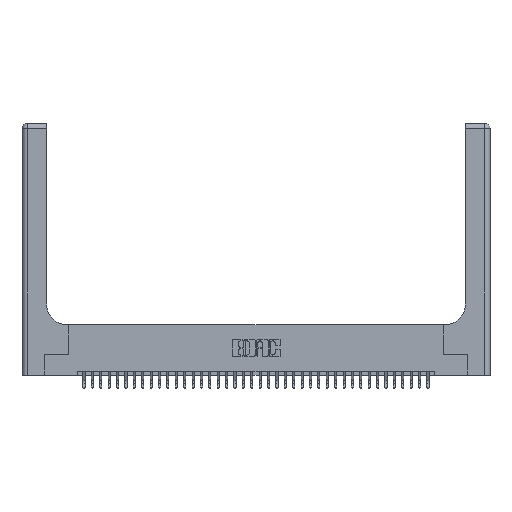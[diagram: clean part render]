
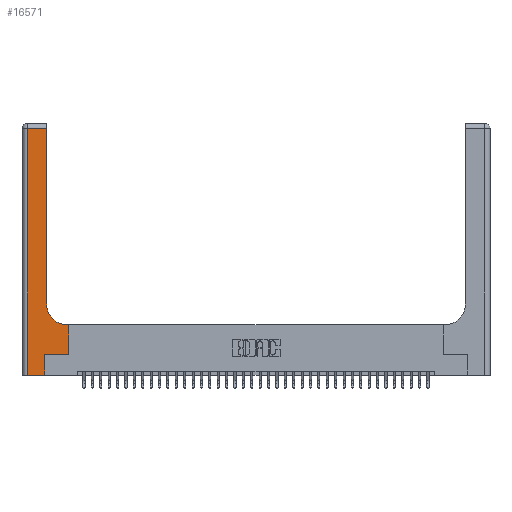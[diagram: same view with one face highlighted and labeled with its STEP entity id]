
A CAD part, top view. The second image highlights one B-rep face of the part: STEP entity #16571.
In plain terms, the highlighted planar face has unit normal (0, 0, 1).
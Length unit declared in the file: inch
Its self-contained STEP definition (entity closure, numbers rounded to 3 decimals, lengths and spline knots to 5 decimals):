
#572 = ORIENTED_EDGE ( 'NONE', *, *, #17456, .T. ) ;
#1190 = CARTESIAN_POINT ( 'NONE',  ( 0.5415, 0.6, 0.37 ) ) ;
#1477 = ORIENTED_EDGE ( 'NONE', *, *, #24891, .T. ) ;
#1787 = VERTEX_POINT ( 'NONE', #2523 ) ;
#2523 = CARTESIAN_POINT ( 'NONE',  ( 0.269, 0.25, 0.37 ) ) ;
#2526 = CARTESIAN_POINT ( 'NONE',  ( 0.2915, 3., 0.37 ) ) ;
#2559 = VERTEX_POINT ( 'NONE', #15699 ) ;
#3589 = DIRECTION ( 'NONE',  ( -1., 0., 0. ) ) ;
#4017 = VERTEX_POINT ( 'NONE', #8633 ) ;
#4109 = CARTESIAN_POINT ( 'NONE',  ( 0., 2.94, 0.37 ) ) ;
#5986 = LINE ( 'NONE', #30661, #36426 ) ;
#6241 = CARTESIAN_POINT ( 'NONE',  ( 0.5585, 0.6, 0.37 ) ) ;
#7123 = DIRECTION ( 'NONE',  ( -1., 0., 0. ) ) ;
#7644 = VECTOR ( 'NONE', #7123, 39.37008 ) ;
#7883 = DIRECTION ( 'NONE',  ( 1., 0., 0. ) ) ;
#7961 = LINE ( 'NONE', #22802, #38336 ) ;
#8111 = DIRECTION ( 'NONE',  ( 0., 0., -1. ) ) ;
#8420 = DIRECTION ( 'NONE',  ( 1., 0., 0. ) ) ;
#8490 = CARTESIAN_POINT ( 'NONE',  ( 0.5585, 0.25, 0.37 ) ) ;
#8607 = ORIENTED_EDGE ( 'NONE', *, *, #38312, .T. ) ;
#8633 = CARTESIAN_POINT ( 'NONE',  ( 0.06, 2.94, 0.37 ) ) ;
#9130 = EDGE_CURVE ( 'NONE', #36194, #2559, #30862, .T. ) ;
#9610 = VERTEX_POINT ( 'NONE', #32164 ) ;
#11884 = CARTESIAN_POINT ( 'NONE',  ( 0.2915, 0.6, 0.37 ) ) ;
#12904 = EDGE_CURVE ( 'NONE', #4017, #34109, #5986, .T. ) ;
#14353 = DIRECTION ( 'NONE',  ( 0., 1., 0. ) ) ;
#14643 = VERTEX_POINT ( 'NONE', #6241 ) ;
#15406 = EDGE_CURVE ( 'NONE', #2559, #4017, #23426, .T. ) ;
#15699 = CARTESIAN_POINT ( 'NONE',  ( 0.2915, 2.94, 0.37 ) ) ;
#16052 = ORIENTED_EDGE ( 'NONE', *, *, #33012, .T. ) ;
#16272 = EDGE_LOOP ( 'NONE', ( #37103, #29817, #30291, #1477, #16052, #33520, #572, #8607, #33026 ) ) ;
#16571 = ADVANCED_FACE ( 'NONE', ( #29490 ), #36013, .F. ) ;
#16711 = CARTESIAN_POINT ( 'NONE',  ( 0., 0., 0.37 ) ) ;
#17456 = EDGE_CURVE ( 'NONE', #27485, #14643, #7961, .T. ) ;
#18151 = CARTESIAN_POINT ( 'NONE',  ( 0.06, 0., 0.37 ) ) ;
#18473 = CARTESIAN_POINT ( 'NONE',  ( 0., 3., 0.37 ) ) ;
#20072 = CARTESIAN_POINT ( 'NONE',  ( 0.2915, 0.85, 0.37 ) ) ;
#21445 = DIRECTION ( 'NONE',  ( 0., 0., -1. ) ) ;
#21608 = EDGE_CURVE ( 'NONE', #30002, #36194, #34286, .T. ) ;
#22577 = AXIS2_PLACEMENT_3D ( 'NONE', #25813, #8111, #28768 ) ;
#22727 = LINE ( 'NONE', #23182, #31421 ) ;
#22802 = CARTESIAN_POINT ( 'NONE',  ( 0.5585, 0.25, 0.37 ) ) ;
#23058 = EDGE_CURVE ( 'NONE', #1787, #27485, #22727, .T. ) ;
#23182 = CARTESIAN_POINT ( 'NONE',  ( 0.269, 0.25, 0.37 ) ) ;
#23386 = DIRECTION ( 'NONE',  ( 0., 1., 0. ) ) ;
#23426 = LINE ( 'NONE', #4109, #7644 ) ;
#23662 = DIRECTION ( 'NONE',  ( -1., 0., 0. ) ) ;
#24891 = EDGE_CURVE ( 'NONE', #34109, #9610, #33944, .T. ) ;
#24895 = DIRECTION ( 'NONE',  ( 0., -1., 0. ) ) ;
#25259 = VECTOR ( 'NONE', #7883, 39.37008 ) ;
#25813 = CARTESIAN_POINT ( 'NONE',  ( 0.5415, 0.85, 0.37 ) ) ;
#27071 = LINE ( 'NONE', #11884, #27974 ) ;
#27485 = VERTEX_POINT ( 'NONE', #8490 ) ;
#27974 = VECTOR ( 'NONE', #23662, 39.37008 ) ;
#28194 = VECTOR ( 'NONE', #14353, 39.37008 ) ;
#28768 = DIRECTION ( 'NONE',  ( 1., 0., 0. ) ) ;
#29044 = CARTESIAN_POINT ( 'NONE',  ( 0.269, 0., 0.37 ) ) ;
#29490 = FACE_OUTER_BOUND ( 'NONE', #16272, .T. ) ;
#29817 = ORIENTED_EDGE ( 'NONE', *, *, #15406, .T. ) ;
#29950 = VECTOR ( 'NONE', #23386, 39.37008 ) ;
#30002 = VERTEX_POINT ( 'NONE', #1190 ) ;
#30291 = ORIENTED_EDGE ( 'NONE', *, *, #12904, .T. ) ;
#30661 = CARTESIAN_POINT ( 'NONE',  ( 0.06, 3., 0.37 ) ) ;
#30862 = LINE ( 'NONE', #2526, #29950 ) ;
#31421 = VECTOR ( 'NONE', #8420, 39.37008 ) ;
#31616 = DIRECTION ( 'NONE',  ( 0., 1., 0. ) ) ;
#32164 = CARTESIAN_POINT ( 'NONE',  ( 0.269, 0., 0.37 ) ) ;
#32782 = AXIS2_PLACEMENT_3D ( 'NONE', #18473, #21445, #3589 ) ;
#33012 = EDGE_CURVE ( 'NONE', #9610, #1787, #37803, .T. ) ;
#33026 = ORIENTED_EDGE ( 'NONE', *, *, #21608, .T. ) ;
#33520 = ORIENTED_EDGE ( 'NONE', *, *, #23058, .T. ) ;
#33944 = LINE ( 'NONE', #16711, #25259 ) ;
#34109 = VERTEX_POINT ( 'NONE', #18151 ) ;
#34286 = CIRCLE ( 'NONE', #22577, 0.25 ) ;
#36013 = PLANE ( 'NONE',  #32782 ) ;
#36194 = VERTEX_POINT ( 'NONE', #20072 ) ;
#36426 = VECTOR ( 'NONE', #24895, 39.37008 ) ;
#37103 = ORIENTED_EDGE ( 'NONE', *, *, #9130, .T. ) ;
#37803 = LINE ( 'NONE', #29044, #28194 ) ;
#38312 = EDGE_CURVE ( 'NONE', #14643, #30002, #27071, .T. ) ;
#38336 = VECTOR ( 'NONE', #31616, 39.37008 ) ;
